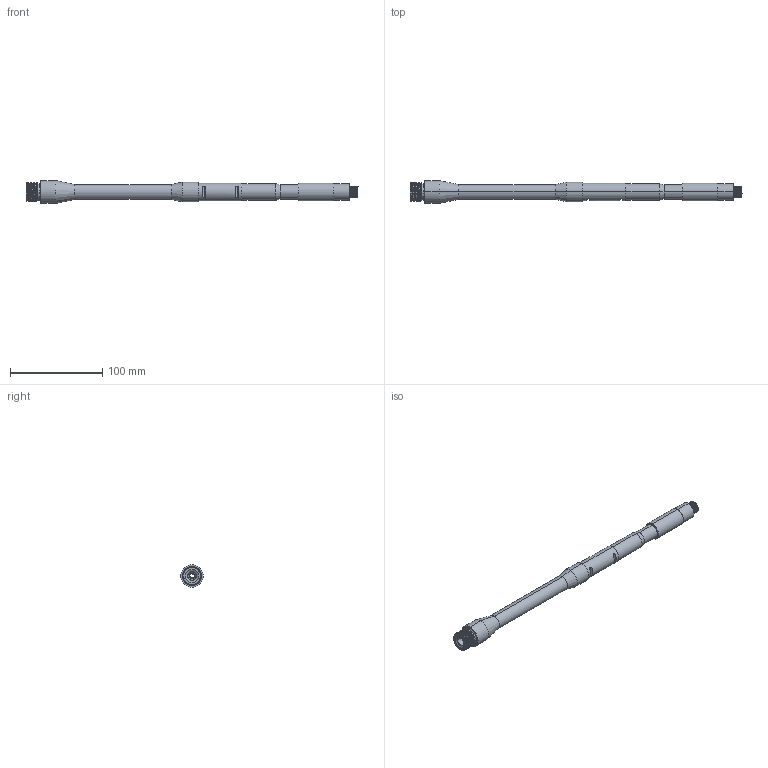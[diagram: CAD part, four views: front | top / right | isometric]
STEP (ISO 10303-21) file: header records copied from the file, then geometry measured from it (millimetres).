
FILE_DESCRIPTION (( 'STEP AP214' ), '1' );
FILE_NAME ('Barrel.step.step', '2019-12-18T03:07:06', ( '' ), ( '' ), 'SwSTEP 2.0', 'SolidWorks 2019', '' );
FILE_SCHEMA (( 'AUTOMOTIVE_DESIGN' ));
Length unit declared in the file: millimetre
Products named in the file (1): Barrel.step
Bounding box: 360.58 x 24.89 x 24.89 mm (x, y, z)
Volume: 84286.9 mm3; surface area: 29334.3 mm2
Topology: 1 solids, 1 shells, 260 faces, 702 edges, 452 vertices
Faces by surface type: cylinder 159, cone 72, bspline 15, plane 10, torus 4
Entity records: 22780 total; most frequent: CARTESIAN_POINT 16914, ORIENTED_EDGE 1404, DIRECTION 930, EDGE_CURVE 702, VERTEX_POINT 452, B_SPLINE_CURVE_WITH_KNOTS 372, AXIS2_PLACEMENT_3D 355, EDGE_LOOP 272
